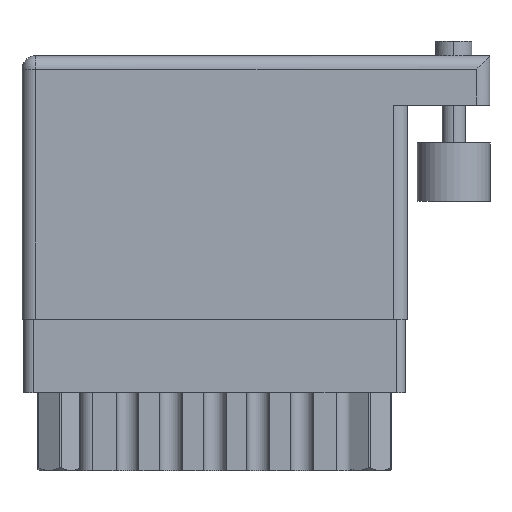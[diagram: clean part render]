
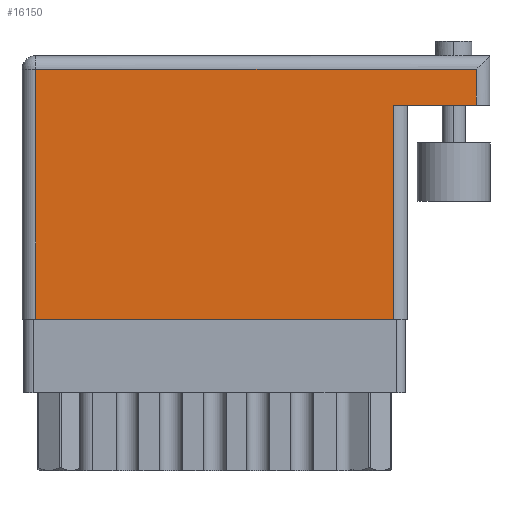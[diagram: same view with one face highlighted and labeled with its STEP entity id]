
A CAD part, front view. The second image highlights one B-rep face of the part: STEP entity #16150.
In plain terms, the highlighted face is planar.
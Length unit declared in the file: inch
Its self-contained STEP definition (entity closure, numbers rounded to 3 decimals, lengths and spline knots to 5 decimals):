
#1074 = AXIS2_PLACEMENT_3D ( 'NONE', #14901, #1572, #22973 ) ;
#1572 = DIRECTION ( 'NONE',  ( 0., 0., -1. ) ) ;
#2930 = DIRECTION ( 'NONE',  ( 0., 1., 0. ) ) ;
#4478 = EDGE_CURVE ( 'NONE', #9788, #18688, #21533, .T. ) ;
#4872 = CARTESIAN_POINT ( 'NONE',  ( 1.562, 0.906, 0. ) ) ;
#4882 = FACE_OUTER_BOUND ( 'NONE', #19458, .T. ) ;
#4915 = EDGE_CURVE ( 'NONE', #19562, #30598, #29512, .T. ) ;
#4984 = VERTEX_POINT ( 'NONE', #10096 ) ;
#5139 = ORIENTED_EDGE ( 'NONE', *, *, #31971, .F. ) ;
#5174 = ORIENTED_EDGE ( 'NONE', *, *, #14136, .T. ) ;
#5357 = DIRECTION ( 'NONE',  ( 1., 0., 0. ) ) ;
#6765 = LINE ( 'NONE', #22904, #32879 ) ;
#6967 = CARTESIAN_POINT ( 'NONE',  ( 0., 0.859, 0. ) ) ;
#7930 = CARTESIAN_POINT ( 'NONE',  ( 1.278, 0.736, 0. ) ) ;
#8291 = VECTOR ( 'NONE', #5357, 39.37008 ) ;
#9788 = VERTEX_POINT ( 'NONE', #13886 ) ;
#10096 = CARTESIAN_POINT ( 'NONE',  ( 1.278, 0.736, 0. ) ) ;
#12621 = ORIENTED_EDGE ( 'NONE', *, *, #4478, .T. ) ;
#13214 = CARTESIAN_POINT ( 'NONE',  ( 1.278, 0., 0. ) ) ;
#13426 = VECTOR ( 'NONE', #23101, 39.37008 ) ;
#13886 = CARTESIAN_POINT ( 'NONE',  ( 1.562, 0.736, 0. ) ) ;
#14136 = EDGE_CURVE ( 'NONE', #30598, #4984, #21278, .T. ) ;
#14901 = CARTESIAN_POINT ( 'NONE',  ( 0., 0.906, 0. ) ) ;
#16150 = ADVANCED_FACE ( 'NONE', ( #4882 ), #30822, .F. ) ;
#16700 = DIRECTION ( 'NONE',  ( 0., 1., 0. ) ) ;
#18343 = CARTESIAN_POINT ( 'NONE',  ( 0., 0., 0. ) ) ;
#18688 = VERTEX_POINT ( 'NONE', #34052 ) ;
#19458 = EDGE_LOOP ( 'NONE', ( #32067, #5174, #5139, #12621, #34154, #20832 ) ) ;
#19562 = VERTEX_POINT ( 'NONE', #26109 ) ;
#20832 = ORIENTED_EDGE ( 'NONE', *, *, #27420, .T. ) ;
#21278 = LINE ( 'NONE', #7930, #25497 ) ;
#21533 = LINE ( 'NONE', #4872, #28963 ) ;
#21553 = LINE ( 'NONE', #26768, #31042 ) ;
#22904 = CARTESIAN_POINT ( 'NONE',  ( 1.609, 0.736, 0. ) ) ;
#22973 = DIRECTION ( 'NONE',  ( -1., 0., 0. ) ) ;
#23081 = VERTEX_POINT ( 'NONE', #32058 ) ;
#23101 = DIRECTION ( 'NONE',  ( -1., 0., 0. ) ) ;
#25497 = VECTOR ( 'NONE', #16700, 39.37008 ) ;
#26109 = CARTESIAN_POINT ( 'NONE',  ( 0.047, 0., 0. ) ) ;
#26768 = CARTESIAN_POINT ( 'NONE',  ( 0.047, 0., 0. ) ) ;
#27122 = DIRECTION ( 'NONE',  ( 0., -1., 0. ) ) ;
#27420 = EDGE_CURVE ( 'NONE', #23081, #19562, #21553, .T. ) ;
#28963 = VECTOR ( 'NONE', #2930, 39.37008 ) ;
#29512 = LINE ( 'NONE', #18343, #8291 ) ;
#30598 = VERTEX_POINT ( 'NONE', #13214 ) ;
#30751 = DIRECTION ( 'NONE',  ( -1., 0., 0. ) ) ;
#30822 = PLANE ( 'NONE',  #1074 ) ;
#31042 = VECTOR ( 'NONE', #27122, 39.37008 ) ;
#31971 = EDGE_CURVE ( 'NONE', #9788, #4984, #6765, .T. ) ;
#32058 = CARTESIAN_POINT ( 'NONE',  ( 0.047, 0.859, 0. ) ) ;
#32067 = ORIENTED_EDGE ( 'NONE', *, *, #4915, .T. ) ;
#32879 = VECTOR ( 'NONE', #30751, 39.37008 ) ;
#33402 = LINE ( 'NONE', #6967, #13426 ) ;
#34052 = CARTESIAN_POINT ( 'NONE',  ( 1.562, 0.859, 0. ) ) ;
#34154 = ORIENTED_EDGE ( 'NONE', *, *, #34615, .T. ) ;
#34615 = EDGE_CURVE ( 'NONE', #18688, #23081, #33402, .T. ) ;
